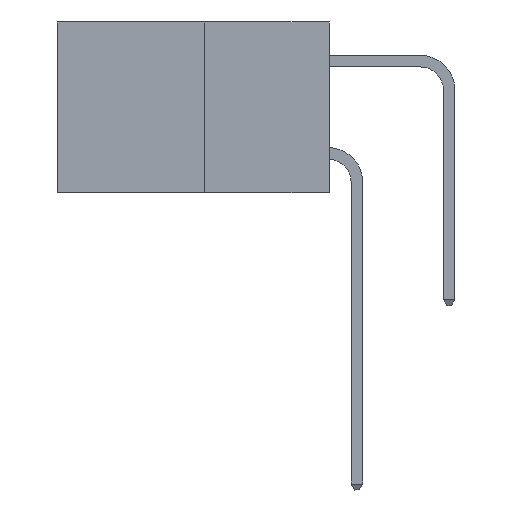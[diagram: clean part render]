
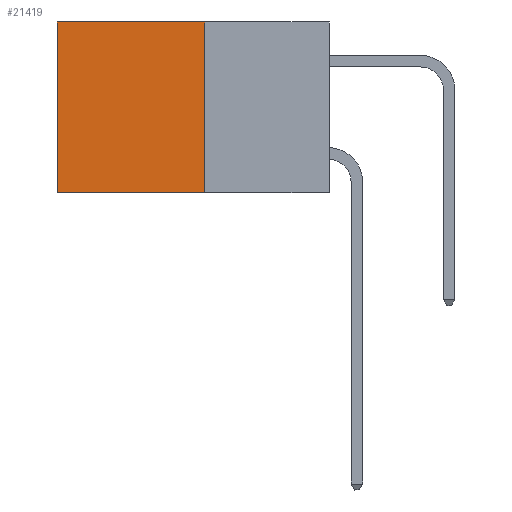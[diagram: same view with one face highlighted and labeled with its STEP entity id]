
A CAD part, left-side view. The second image highlights one B-rep face of the part: STEP entity #21419.
In plain terms, the highlighted planar face has unit normal (-1, 0, 0).
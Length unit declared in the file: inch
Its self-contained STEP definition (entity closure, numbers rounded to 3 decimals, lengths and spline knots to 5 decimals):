
#2238 = VECTOR ( 'NONE', #23369, 39.37008 ) ;
#2581 = LINE ( 'NONE', #19257, #19342 ) ;
#3043 = CARTESIAN_POINT ( 'NONE',  ( 0.277, 0.27, 0. ) ) ;
#3990 = ORIENTED_EDGE ( 'NONE', *, *, #18356, .F. ) ;
#4015 = AXIS2_PLACEMENT_3D ( 'NONE', #5559, #20723, #7793 ) ;
#4786 = CARTESIAN_POINT ( 'NONE',  ( 0.277, 0.27, -0.37 ) ) ;
#5559 = CARTESIAN_POINT ( 'NONE',  ( 0.277, 0.27, -0.37 ) ) ;
#5687 = ORIENTED_EDGE ( 'NONE', *, *, #12479, .T. ) ;
#7190 = EDGE_CURVE ( 'NONE', #10878, #13471, #11267, .T. ) ;
#7536 = DIRECTION ( 'NONE',  ( 0., 1., 0. ) ) ;
#7793 = DIRECTION ( 'NONE',  ( 0., 0., -1. ) ) ;
#7986 = ORIENTED_EDGE ( 'NONE', *, *, #7190, .T. ) ;
#8155 = LINE ( 'NONE', #14874, #2238 ) ;
#8455 = DIRECTION ( 'NONE',  ( 0., 0., -1. ) ) ;
#9901 = LINE ( 'NONE', #3043, #26799 ) ;
#9985 = VERTEX_POINT ( 'NONE', #4786 ) ;
#10191 = CARTESIAN_POINT ( 'NONE',  ( 0.277, 0.27, 0. ) ) ;
#10878 = VERTEX_POINT ( 'NONE', #16502 ) ;
#11267 = LINE ( 'NONE', #19256, #21998 ) ;
#12479 = EDGE_CURVE ( 'NONE', #13327, #10878, #9901, .T. ) ;
#12764 = EDGE_CURVE ( 'NONE', #9985, #13471, #8155, .T. ) ;
#13327 = VERTEX_POINT ( 'NONE', #10191 ) ;
#13471 = VERTEX_POINT ( 'NONE', #15019 ) ;
#13683 = ORIENTED_EDGE ( 'NONE', *, *, #12764, .F. ) ;
#14874 = CARTESIAN_POINT ( 'NONE',  ( 0.277, 0.27, -0.37 ) ) ;
#15019 = CARTESIAN_POINT ( 'NONE',  ( 0.277, 0.59, -0.37 ) ) ;
#15167 = FACE_OUTER_BOUND ( 'NONE', #23093, .T. ) ;
#16502 = CARTESIAN_POINT ( 'NONE',  ( 0.277, 0.59, 0. ) ) ;
#17779 = DIRECTION ( 'NONE',  ( 0., 0., -1. ) ) ;
#18356 = EDGE_CURVE ( 'NONE', #13327, #9985, #2581, .T. ) ;
#18610 = PLANE ( 'NONE',  #4015 ) ;
#19256 = CARTESIAN_POINT ( 'NONE',  ( 0.277, 0.59, -0.37 ) ) ;
#19257 = CARTESIAN_POINT ( 'NONE',  ( 0.277, 0.27, -0.37 ) ) ;
#19342 = VECTOR ( 'NONE', #8455, 39.37008 ) ;
#20723 = DIRECTION ( 'NONE',  ( 1., 0., 0. ) ) ;
#21419 = ADVANCED_FACE ( 'NONE', ( #15167 ), #18610, .F. ) ;
#21998 = VECTOR ( 'NONE', #17779, 39.37008 ) ;
#23093 = EDGE_LOOP ( 'NONE', ( #7986, #13683, #3990, #5687 ) ) ;
#23369 = DIRECTION ( 'NONE',  ( 0., 1., 0. ) ) ;
#26799 = VECTOR ( 'NONE', #7536, 39.37008 ) ;
